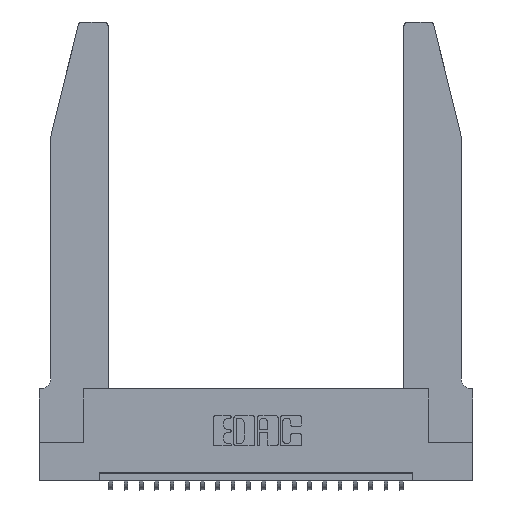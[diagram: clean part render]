
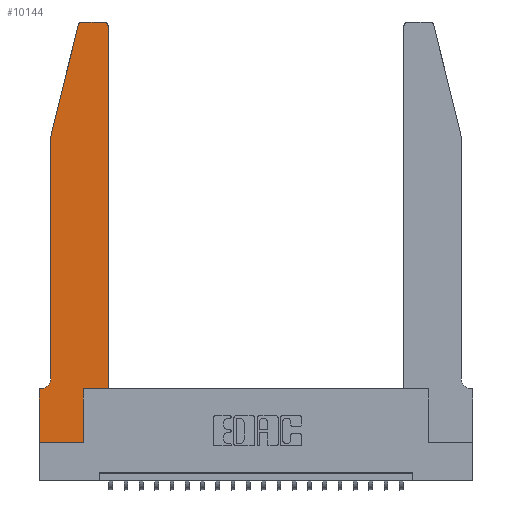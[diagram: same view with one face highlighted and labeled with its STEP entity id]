
A CAD part, top view. The second image highlights one B-rep face of the part: STEP entity #10144.
In plain terms, the highlighted planar face has unit normal (0, 0, 1).
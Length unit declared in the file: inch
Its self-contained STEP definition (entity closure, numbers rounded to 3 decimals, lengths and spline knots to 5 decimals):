
#94 = CARTESIAN_POINT ( 'NONE',  ( 0.0755, 0.35, 0.37 ) ) ;
#460 = EDGE_CURVE ( 'NONE', #14606, #8356, #13161, .T. ) ;
#533 = EDGE_CURVE ( 'NONE', #13091, #21210, #5990, .T. ) ;
#1223 = ORIENTED_EDGE ( 'NONE', *, *, #5603, .T. ) ;
#1269 = CARTESIAN_POINT ( 'NONE',  ( 0.4505, 0.35, 0.37 ) ) ;
#1368 = CARTESIAN_POINT ( 'NONE',  ( 0.0055, 0.35, 0.37 ) ) ;
#1506 = ORIENTED_EDGE ( 'NONE', *, *, #9038, .T. ) ;
#1572 = DIRECTION ( 'NONE',  ( 1., 0., 0. ) ) ;
#1810 = LINE ( 'NONE', #5982, #3450 ) ;
#2137 = AXIS2_PLACEMENT_3D ( 'NONE', #3795, #5587, #10919 ) ;
#2345 = EDGE_CURVE ( 'NONE', #22017, #15636, #16968, .T. ) ;
#2969 = ORIENTED_EDGE ( 'NONE', *, *, #533, .T. ) ;
#2991 = CARTESIAN_POINT ( 'NONE',  ( 0.2865, 0.35, 0.37 ) ) ;
#3450 = VECTOR ( 'NONE', #13157, 39.37008 ) ;
#3795 = CARTESIAN_POINT ( 'NONE',  ( 0.0055, 0.42, 0.37 ) ) ;
#3945 = DIRECTION ( 'NONE',  ( -1., 0., 0. ) ) ;
#4062 = DIRECTION ( 'NONE',  ( 1., 0., 0. ) ) ;
#4105 = EDGE_CURVE ( 'NONE', #6458, #9368, #9456, .T. ) ;
#4859 = CARTESIAN_POINT ( 'NONE',  ( 0.2865, 0.35, 0.37 ) ) ;
#4869 = CARTESIAN_POINT ( 'NONE',  ( 0., 0., 0.37 ) ) ;
#5354 = CARTESIAN_POINT ( 'NONE',  ( 0.284, 2.72, 0.37 ) ) ;
#5547 = CARTESIAN_POINT ( 'NONE',  ( 0.0755, 2., 0.37 ) ) ;
#5549 = LINE ( 'NONE', #20334, #19944 ) ;
#5587 = DIRECTION ( 'NONE',  ( 0., 0., -1. ) ) ;
#5603 = EDGE_CURVE ( 'NONE', #15636, #13091, #15722, .T. ) ;
#5805 = EDGE_CURVE ( 'NONE', #8670, #22484, #14603, .T. ) ;
#5814 = CARTESIAN_POINT ( 'NONE',  ( 0.2605, 2.75, 0.37 ) ) ;
#5982 = CARTESIAN_POINT ( 'NONE',  ( 0.4505, 0.35, 0.37 ) ) ;
#5990 = LINE ( 'NONE', #5547, #14265 ) ;
#6049 = CIRCLE ( 'NONE', #2137, 0.07 ) ;
#6458 = VERTEX_POINT ( 'NONE', #21235 ) ;
#6649 = CARTESIAN_POINT ( 'NONE',  ( 0., 0., 0.37 ) ) ;
#6878 = DIRECTION ( 'NONE',  ( 0., 1., 0. ) ) ;
#8356 = VERTEX_POINT ( 'NONE', #2991 ) ;
#8377 = EDGE_CURVE ( 'NONE', #22484, #21239, #19330, .T. ) ;
#8670 = VERTEX_POINT ( 'NONE', #1269 ) ;
#9038 = EDGE_CURVE ( 'NONE', #21210, #10855, #6049, .T. ) ;
#9368 = VERTEX_POINT ( 'NONE', #4869 ) ;
#9456 = LINE ( 'NONE', #6649, #16612 ) ;
#9753 = ORIENTED_EDGE ( 'NONE', *, *, #8377, .T. ) ;
#10144 = ADVANCED_FACE ( 'NONE', ( #20889 ), #21502, .T. ) ;
#10261 = DIRECTION ( 'NONE',  ( 0., 0., 1. ) ) ;
#10588 = LINE ( 'NONE', #5814, #16949 ) ;
#10855 = VERTEX_POINT ( 'NONE', #1368 ) ;
#10919 = DIRECTION ( 'NONE',  ( -1., 0., 0. ) ) ;
#10931 = ORIENTED_EDGE ( 'NONE', *, *, #5805, .T. ) ;
#11063 = CARTESIAN_POINT ( 'NONE',  ( 0.4205, 2.75, 0.37 ) ) ;
#12217 = DIRECTION ( 'NONE',  ( 1., 0., 0. ) ) ;
#12884 = ORIENTED_EDGE ( 'NONE', *, *, #13745, .T. ) ;
#12965 = EDGE_CURVE ( 'NONE', #21239, #22017, #10588, .T. ) ;
#13003 = ORIENTED_EDGE ( 'NONE', *, *, #4105, .T. ) ;
#13076 = CARTESIAN_POINT ( 'NONE',  ( 0.0755, 0.42, 0.37 ) ) ;
#13091 = VERTEX_POINT ( 'NONE', #21085 ) ;
#13157 = DIRECTION ( 'NONE',  ( 1., 0., 0. ) ) ;
#13161 = LINE ( 'NONE', #4859, #18416 ) ;
#13199 = DIRECTION ( 'NONE',  ( 0., 0., 1. ) ) ;
#13308 = CARTESIAN_POINT ( 'NONE',  ( 0.2865, 0., 0.37 ) ) ;
#13512 = CARTESIAN_POINT ( 'NONE',  ( 0.284, 2.75, 0.37 ) ) ;
#13745 = EDGE_CURVE ( 'NONE', #9368, #14606, #5549, .T. ) ;
#14048 = DIRECTION ( 'NONE',  ( -1., 0., 0. ) ) ;
#14265 = VECTOR ( 'NONE', #17901, 39.37008 ) ;
#14442 = DIRECTION ( 'NONE',  ( -0.239, -0.971, 0. ) ) ;
#14603 = LINE ( 'NONE', #19308, #14905 ) ;
#14606 = VERTEX_POINT ( 'NONE', #13308 ) ;
#14623 = AXIS2_PLACEMENT_3D ( 'NONE', #5354, #10261, #12217 ) ;
#14661 = EDGE_CURVE ( 'NONE', #8356, #8670, #1810, .T. ) ;
#14687 = EDGE_LOOP ( 'NONE', ( #18290, #15230, #1223, #2969, #1506, #22234, #13003, #12884, #22826, #20420, #10931, #9753 ) ) ;
#14905 = VECTOR ( 'NONE', #17752, 39.37008 ) ;
#15020 = CARTESIAN_POINT ( 'NONE',  ( 0.4505, 2.72, 0.37 ) ) ;
#15230 = ORIENTED_EDGE ( 'NONE', *, *, #2345, .T. ) ;
#15636 = VERTEX_POINT ( 'NONE', #17178 ) ;
#15722 = LINE ( 'NONE', #20922, #19893 ) ;
#16268 = DIRECTION ( 'NONE',  ( 0., 0., 1. ) ) ;
#16612 = VECTOR ( 'NONE', #19227, 39.37008 ) ;
#16949 = VECTOR ( 'NONE', #3945, 39.37008 ) ;
#16968 = CIRCLE ( 'NONE', #14623, 0.03 ) ;
#17135 = VECTOR ( 'NONE', #14048, 39.37008 ) ;
#17178 = CARTESIAN_POINT ( 'NONE',  ( 0.25487, 2.72718, 0.37 ) ) ;
#17752 = DIRECTION ( 'NONE',  ( 0., 1., 0. ) ) ;
#17901 = DIRECTION ( 'NONE',  ( 0., -1., 0. ) ) ;
#18290 = ORIENTED_EDGE ( 'NONE', *, *, #12965, .T. ) ;
#18416 = VECTOR ( 'NONE', #6878, 39.37008 ) ;
#18614 = AXIS2_PLACEMENT_3D ( 'NONE', #19844, #13199, #4062 ) ;
#18734 = EDGE_CURVE ( 'NONE', #10855, #6458, #21811, .T. ) ;
#19227 = DIRECTION ( 'NONE',  ( 0., -1., 0. ) ) ;
#19308 = CARTESIAN_POINT ( 'NONE',  ( 0.4505, 0.35, 0.37 ) ) ;
#19330 = CIRCLE ( 'NONE', #20216, 0.03 ) ;
#19844 = CARTESIAN_POINT ( 'NONE',  ( 0., 0.35, 0.37 ) ) ;
#19893 = VECTOR ( 'NONE', #14442, 39.37008 ) ;
#19944 = VECTOR ( 'NONE', #21689, 39.37008 ) ;
#20216 = AXIS2_PLACEMENT_3D ( 'NONE', #22616, #16268, #1572 ) ;
#20334 = CARTESIAN_POINT ( 'NONE',  ( 0., 0., 0.37 ) ) ;
#20420 = ORIENTED_EDGE ( 'NONE', *, *, #14661, .T. ) ;
#20889 = FACE_OUTER_BOUND ( 'NONE', #14687, .T. ) ;
#20922 = CARTESIAN_POINT ( 'NONE',  ( 0.0755, 2., 0.37 ) ) ;
#21085 = CARTESIAN_POINT ( 'NONE',  ( 0.0755, 2., 0.37 ) ) ;
#21210 = VERTEX_POINT ( 'NONE', #13076 ) ;
#21235 = CARTESIAN_POINT ( 'NONE',  ( 0., 0.35, 0.37 ) ) ;
#21239 = VERTEX_POINT ( 'NONE', #11063 ) ;
#21502 = PLANE ( 'NONE',  #18614 ) ;
#21689 = DIRECTION ( 'NONE',  ( 1., 0., 0. ) ) ;
#21811 = LINE ( 'NONE', #94, #17135 ) ;
#22017 = VERTEX_POINT ( 'NONE', #13512 ) ;
#22234 = ORIENTED_EDGE ( 'NONE', *, *, #18734, .T. ) ;
#22484 = VERTEX_POINT ( 'NONE', #15020 ) ;
#22616 = CARTESIAN_POINT ( 'NONE',  ( 0.4205, 2.72, 0.37 ) ) ;
#22826 = ORIENTED_EDGE ( 'NONE', *, *, #460, .T. ) ;
